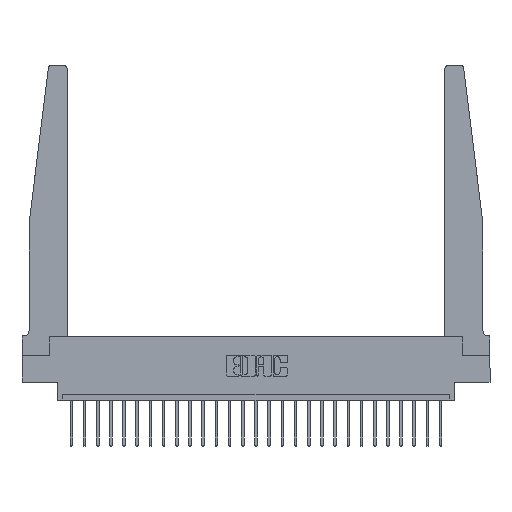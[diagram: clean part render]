
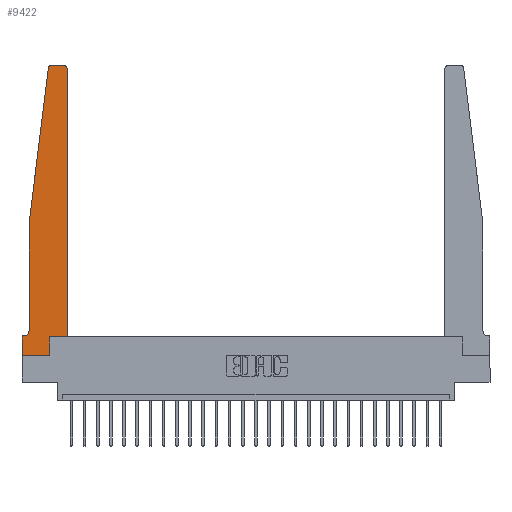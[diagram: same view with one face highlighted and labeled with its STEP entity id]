
A CAD part, top view. The second image highlights one B-rep face of the part: STEP entity #9422.
In plain terms, the highlighted planar face has unit normal (0, 0, 1).
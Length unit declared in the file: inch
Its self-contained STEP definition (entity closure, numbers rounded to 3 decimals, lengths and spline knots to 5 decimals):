
#500 = CARTESIAN_POINT ( 'NONE',  ( 0., 0.1875, 0.37 ) ) ;
#1532 = AXIS2_PLACEMENT_3D ( 'NONE', #3531, #11143, #24620 ) ;
#1893 = VERTEX_POINT ( 'NONE', #9783 ) ;
#2145 = EDGE_CURVE ( 'NONE', #14729, #11471, #9490, .T. ) ;
#2238 = CARTESIAN_POINT ( 'NONE',  ( 0.2605, 0.18, 0.37 ) ) ;
#2549 = LINE ( 'NONE', #22372, #8006 ) ;
#3158 = PLANE ( 'NONE',  #1532 ) ;
#3531 = CARTESIAN_POINT ( 'NONE',  ( 0., 0.1875, 0.37 ) ) ;
#3639 = CIRCLE ( 'NONE', #18672, 0.03 ) ;
#3656 = CARTESIAN_POINT ( 'NONE',  ( 0.24675, 2.72367, 0.37 ) ) ;
#3711 = VECTOR ( 'NONE', #10019, 39.37008 ) ;
#4439 = CARTESIAN_POINT ( 'NONE',  ( 0.015, 0.1875, 0.37 ) ) ;
#4526 = DIRECTION ( 'NONE',  ( -1., 0., 0. ) ) ;
#4827 = EDGE_CURVE ( 'NONE', #7830, #5367, #19685, .T. ) ;
#4926 = ORIENTED_EDGE ( 'NONE', *, *, #19229, .T. ) ;
#4933 = DIRECTION ( 'NONE',  ( 1., 0., 0. ) ) ;
#4981 = CARTESIAN_POINT ( 'NONE',  ( 0.27653, 2.75, 0.37 ) ) ;
#5072 = CARTESIAN_POINT ( 'NONE',  ( 0.2605, 0., 0.37 ) ) ;
#5334 = DIRECTION ( 'NONE',  ( 0., 0., -1. ) ) ;
#5367 = VERTEX_POINT ( 'NONE', #2238 ) ;
#5570 = CARTESIAN_POINT ( 'NONE',  ( 0.015, 0.2375, 0.37 ) ) ;
#5636 = EDGE_CURVE ( 'NONE', #14968, #14875, #16536, .T. ) ;
#6197 = DIRECTION ( 'NONE',  ( 0., 1., 0. ) ) ;
#6897 = DIRECTION ( 'NONE',  ( 0., 0., 1. ) ) ;
#7280 = EDGE_CURVE ( 'NONE', #12222, #17002, #17750, .T. ) ;
#7494 = CARTESIAN_POINT ( 'NONE',  ( 0.065, 1.25, 0.37 ) ) ;
#7594 = AXIS2_PLACEMENT_3D ( 'NONE', #20639, #6897, #8930 ) ;
#7759 = DIRECTION ( 'NONE',  ( -1., 0., 0. ) ) ;
#7830 = VERTEX_POINT ( 'NONE', #5072 ) ;
#8006 = VECTOR ( 'NONE', #4933, 39.37008 ) ;
#8306 = ORIENTED_EDGE ( 'NONE', *, *, #2145, .T. ) ;
#8360 = CARTESIAN_POINT ( 'NONE',  ( 0., 0., 0.37 ) ) ;
#8365 = VECTOR ( 'NONE', #6197, 39.37008 ) ;
#8675 = DIRECTION ( 'NONE',  ( 1., 0., 0. ) ) ;
#8930 = DIRECTION ( 'NONE',  ( 1., 0., 0. ) ) ;
#9047 = EDGE_CURVE ( 'NONE', #17002, #14968, #18714, .T. ) ;
#9175 = EDGE_CURVE ( 'NONE', #13836, #14143, #14084, .T. ) ;
#9264 = DIRECTION ( 'NONE',  ( -1., 0., 0. ) ) ;
#9276 = DIRECTION ( 'NONE',  ( -0.122, -0.992, 0. ) ) ;
#9372 = EDGE_CURVE ( 'NONE', #5367, #14729, #2549, .T. ) ;
#9422 = ADVANCED_FACE ( 'NONE', ( #24760 ), #3158, .T. ) ;
#9490 = LINE ( 'NONE', #14847, #19023 ) ;
#9783 = CARTESIAN_POINT ( 'NONE',  ( 0.395, 2.75, 0.37 ) ) ;
#10019 = DIRECTION ( 'NONE',  ( 1., 0., 0. ) ) ;
#10241 = LINE ( 'NONE', #18008, #16954 ) ;
#10640 = CARTESIAN_POINT ( 'NONE',  ( 0., 0., 0.37 ) ) ;
#11143 = DIRECTION ( 'NONE',  ( 0., 0., 1. ) ) ;
#11373 = AXIS2_PLACEMENT_3D ( 'NONE', #5570, #5334, #9264 ) ;
#11471 = VERTEX_POINT ( 'NONE', #23219 ) ;
#11647 = VECTOR ( 'NONE', #12328, 39.37008 ) ;
#11934 = ORIENTED_EDGE ( 'NONE', *, *, #9047, .T. ) ;
#12168 = LINE ( 'NONE', #10640, #24786 ) ;
#12222 = VERTEX_POINT ( 'NONE', #4981 ) ;
#12328 = DIRECTION ( 'NONE',  ( 0., -1., 0. ) ) ;
#12741 = EDGE_CURVE ( 'NONE', #14875, #13836, #21134, .T. ) ;
#13374 = ORIENTED_EDGE ( 'NONE', *, *, #22416, .T. ) ;
#13433 = EDGE_LOOP ( 'NONE', ( #19659, #18803, #11934, #22616, #20019, #13801, #13374, #13908, #24555, #20503, #8306, #4926 ) ) ;
#13700 = CARTESIAN_POINT ( 'NONE',  ( 0.2605, 0.18, 0.37 ) ) ;
#13801 = ORIENTED_EDGE ( 'NONE', *, *, #9175, .T. ) ;
#13836 = VERTEX_POINT ( 'NONE', #4439 ) ;
#13877 = EDGE_CURVE ( 'NONE', #21225, #7830, #23639, .T. ) ;
#13908 = ORIENTED_EDGE ( 'NONE', *, *, #13877, .T. ) ;
#14084 = LINE ( 'NONE', #17930, #15327 ) ;
#14143 = VERTEX_POINT ( 'NONE', #500 ) ;
#14534 = DIRECTION ( 'NONE',  ( 0., 0., 1. ) ) ;
#14728 = DIRECTION ( 'NONE',  ( 0., 1., 0. ) ) ;
#14729 = VERTEX_POINT ( 'NONE', #20616 ) ;
#14782 = CARTESIAN_POINT ( 'NONE',  ( 0.395, 2.72, 0.37 ) ) ;
#14847 = CARTESIAN_POINT ( 'NONE',  ( 0.425, 0.18, 0.37 ) ) ;
#14875 = VERTEX_POINT ( 'NONE', #19600 ) ;
#14968 = VERTEX_POINT ( 'NONE', #19337 ) ;
#15327 = VECTOR ( 'NONE', #7759, 39.37008 ) ;
#16415 = CARTESIAN_POINT ( 'NONE',  ( 0.065, 1.25, 0.37 ) ) ;
#16536 = LINE ( 'NONE', #16415, #11647 ) ;
#16954 = VECTOR ( 'NONE', #4526, 39.37008 ) ;
#17002 = VERTEX_POINT ( 'NONE', #3656 ) ;
#17750 = CIRCLE ( 'NONE', #7594, 0.03 ) ;
#17919 = DIRECTION ( 'NONE',  ( 0., -1., 0. ) ) ;
#17930 = CARTESIAN_POINT ( 'NONE',  ( 0.065, 0.1875, 0.37 ) ) ;
#18008 = CARTESIAN_POINT ( 'NONE',  ( 0.25, 2.75, 0.37 ) ) ;
#18672 = AXIS2_PLACEMENT_3D ( 'NONE', #14782, #14534, #8675 ) ;
#18714 = LINE ( 'NONE', #7494, #21062 ) ;
#18803 = ORIENTED_EDGE ( 'NONE', *, *, #7280, .T. ) ;
#19023 = VECTOR ( 'NONE', #14728, 39.37008 ) ;
#19229 = EDGE_CURVE ( 'NONE', #11471, #1893, #3639, .T. ) ;
#19337 = CARTESIAN_POINT ( 'NONE',  ( 0.065, 1.25, 0.37 ) ) ;
#19600 = CARTESIAN_POINT ( 'NONE',  ( 0.065, 0.2375, 0.37 ) ) ;
#19659 = ORIENTED_EDGE ( 'NONE', *, *, #23950, .T. ) ;
#19685 = LINE ( 'NONE', #13700, #8365 ) ;
#20019 = ORIENTED_EDGE ( 'NONE', *, *, #12741, .T. ) ;
#20503 = ORIENTED_EDGE ( 'NONE', *, *, #9372, .T. ) ;
#20616 = CARTESIAN_POINT ( 'NONE',  ( 0.425, 0.18, 0.37 ) ) ;
#20639 = CARTESIAN_POINT ( 'NONE',  ( 0.27653, 2.72, 0.37 ) ) ;
#21062 = VECTOR ( 'NONE', #9276, 39.37008 ) ;
#21134 = CIRCLE ( 'NONE', #11373, 0.05 ) ;
#21225 = VERTEX_POINT ( 'NONE', #23888 ) ;
#22372 = CARTESIAN_POINT ( 'NONE',  ( 0.425, 0.18, 0.37 ) ) ;
#22416 = EDGE_CURVE ( 'NONE', #14143, #21225, #12168, .T. ) ;
#22616 = ORIENTED_EDGE ( 'NONE', *, *, #5636, .T. ) ;
#23219 = CARTESIAN_POINT ( 'NONE',  ( 0.425, 2.72, 0.37 ) ) ;
#23639 = LINE ( 'NONE', #8360, #3711 ) ;
#23888 = CARTESIAN_POINT ( 'NONE',  ( 0., 0., 0.37 ) ) ;
#23950 = EDGE_CURVE ( 'NONE', #1893, #12222, #10241, .T. ) ;
#24555 = ORIENTED_EDGE ( 'NONE', *, *, #4827, .T. ) ;
#24620 = DIRECTION ( 'NONE',  ( 1., 0., 0. ) ) ;
#24760 = FACE_OUTER_BOUND ( 'NONE', #13433, .T. ) ;
#24786 = VECTOR ( 'NONE', #17919, 39.37008 ) ;
